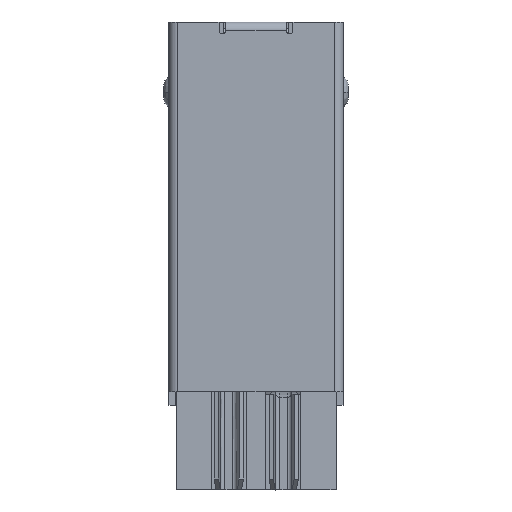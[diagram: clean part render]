
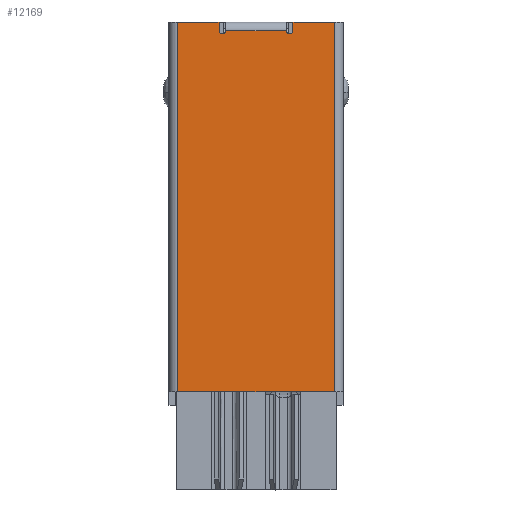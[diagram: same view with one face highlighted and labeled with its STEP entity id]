
A CAD part, front view. The second image highlights one B-rep face of the part: STEP entity #12169.
In plain terms, the highlighted face is planar.
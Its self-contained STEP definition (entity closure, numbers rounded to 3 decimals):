
#36 = CARTESIAN_POINT ( 'NONE',  ( 15.775, 8.618, 0. ) ) ;
#47 = CARTESIAN_POINT ( 'NONE',  ( 15.775, 13.918, -17. ) ) ;
#470 = CARTESIAN_POINT ( 'NONE',  ( 15.775, 12.018, -0.4 ) ) ;
#772 = EDGE_CURVE ( 'NONE', #9003, #23572, #12551, .T. ) ;
#1052 = CARTESIAN_POINT ( 'NONE',  ( 15.775, 10.318, 0. ) ) ;
#1074 = DIRECTION ( 'NONE',  ( -1., 0., 0. ) ) ;
#1161 = VERTEX_POINT ( 'NONE', #36 ) ;
#1164 = DIRECTION ( 'NONE',  ( -1., 0., 0. ) ) ;
#1390 = CARTESIAN_POINT ( 'NONE',  ( 15.775, 10.318, -17. ) ) ;
#1419 = ORIENTED_EDGE ( 'NONE', *, *, #16090, .T. ) ;
#1442 = AXIS2_PLACEMENT_3D ( 'NONE', #2475, #9698, #9934 ) ;
#1840 = DIRECTION ( 'NONE',  ( 1., 0., 0. ) ) ;
#1901 = DIRECTION ( 'NONE',  ( 0., 0., 1. ) ) ;
#1944 = CARTESIAN_POINT ( 'NONE',  ( 15.775, 6.718, -17. ) ) ;
#2215 = CARTESIAN_POINT ( 'NONE',  ( 15.775, 11.718, -0.4 ) ) ;
#2237 = LINE ( 'NONE', #2469, #21916 ) ;
#2265 = EDGE_LOOP ( 'NONE', ( #2969, #20408, #13631, #16832, #23114, #19453, #1419, #18053, #5312, #18673, #3849 ) ) ;
#2469 = CARTESIAN_POINT ( 'NONE',  ( 15.775, 10.318, -0.4 ) ) ;
#2475 = CARTESIAN_POINT ( 'NONE',  ( 15.775, 8.768, -0.4 ) ) ;
#2521 = DIRECTION ( 'NONE',  ( 0., -1., 0. ) ) ;
#2943 = CIRCLE ( 'NONE', #11157, 0.15 ) ;
#2969 = ORIENTED_EDGE ( 'NONE', *, *, #10550, .T. ) ;
#3849 = ORIENTED_EDGE ( 'NONE', *, *, #772, .T. ) ;
#4062 = CARTESIAN_POINT ( 'NONE',  ( 15.775, 6.718, 0. ) ) ;
#4131 = VERTEX_POINT ( 'NONE', #4062 ) ;
#5312 = ORIENTED_EDGE ( 'NONE', *, *, #13490, .T. ) ;
#5510 = CARTESIAN_POINT ( 'NONE',  ( 15.775, 6.568, -17.34 ) ) ;
#5815 = DIRECTION ( 'NONE',  ( 0., -1., 0. ) ) ;
#5989 = LINE ( 'NONE', #21129, #10350 ) ;
#6026 = DIRECTION ( 'NONE',  ( 0., -1., 0. ) ) ;
#6603 = EDGE_CURVE ( 'NONE', #22837, #13406, #2237, .T. ) ;
#6836 = AXIS2_PLACEMENT_3D ( 'NONE', #5510, #1840, #20425 ) ;
#6957 = DIRECTION ( 'NONE',  ( 0., 0., -1. ) ) ;
#7524 = EDGE_CURVE ( 'NONE', #21840, #1161, #18659, .T. ) ;
#7940 = CARTESIAN_POINT ( 'NONE',  ( 15.775, 8.918, -0.4 ) ) ;
#8231 = CARTESIAN_POINT ( 'NONE',  ( 15.775, 6.718, -8.5 ) ) ;
#9003 = VERTEX_POINT ( 'NONE', #9581 ) ;
#9063 = PLANE ( 'NONE',  #6836 ) ;
#9328 = LINE ( 'NONE', #1390, #12747 ) ;
#9367 = VERTEX_POINT ( 'NONE', #14322 ) ;
#9581 = CARTESIAN_POINT ( 'NONE',  ( 15.775, 12.018, 0. ) ) ;
#9698 = DIRECTION ( 'NONE',  ( -1., 0., 0. ) ) ;
#9724 = LINE ( 'NONE', #9962, #23338 ) ;
#9934 = DIRECTION ( 'NONE',  ( 0., 0., -1. ) ) ;
#9962 = CARTESIAN_POINT ( 'NONE',  ( 15.775, 10.318, 0. ) ) ;
#10094 = DIRECTION ( 'NONE',  ( 0., 0., 1. ) ) ;
#10123 = EDGE_CURVE ( 'NONE', #13406, #21769, #15832, .T. ) ;
#10350 = VECTOR ( 'NONE', #13458, 1000. ) ;
#10550 = EDGE_CURVE ( 'NONE', #23572, #22837, #2943, .T. ) ;
#10589 = CARTESIAN_POINT ( 'NONE',  ( 15.775, 11.868, -0.4 ) ) ;
#10834 = VERTEX_POINT ( 'NONE', #47 ) ;
#11126 = VERTEX_POINT ( 'NONE', #1944 ) ;
#11157 = AXIS2_PLACEMENT_3D ( 'NONE', #10589, #1164, #10094 ) ;
#11193 = CARTESIAN_POINT ( 'NONE',  ( 15.775, 8.618, -8.5 ) ) ;
#12169 = ADVANCED_FACE ( 'NONE', ( #12855 ), #9063, .T. ) ;
#12551 = LINE ( 'NONE', #14519, #22301 ) ;
#12747 = VECTOR ( 'NONE', #19978, 1000. ) ;
#12759 = VECTOR ( 'NONE', #19605, 1000. ) ;
#12855 = FACE_OUTER_BOUND ( 'NONE', #2265, .T. ) ;
#13406 = VERTEX_POINT ( 'NONE', #7940 ) ;
#13458 = DIRECTION ( 'NONE',  ( 0., 0., 1. ) ) ;
#13490 = EDGE_CURVE ( 'NONE', #10834, #9367, #5989, .T. ) ;
#13631 = ORIENTED_EDGE ( 'NONE', *, *, #10123, .T. ) ;
#13873 = EDGE_CURVE ( 'NONE', #1161, #4131, #17942, .T. ) ;
#13991 = LINE ( 'NONE', #8231, #12759 ) ;
#14322 = CARTESIAN_POINT ( 'NONE',  ( 15.775, 13.918, 0. ) ) ;
#14416 = CARTESIAN_POINT ( 'NONE',  ( 15.775, 8.768, -0.4 ) ) ;
#14519 = CARTESIAN_POINT ( 'NONE',  ( 15.775, 12.018, -8.5 ) ) ;
#15832 = CIRCLE ( 'NONE', #20953, 0.15 ) ;
#16090 = EDGE_CURVE ( 'NONE', #4131, #11126, #13991, .T. ) ;
#16832 = ORIENTED_EDGE ( 'NONE', *, *, #20488, .T. ) ;
#17942 = LINE ( 'NONE', #1052, #18576 ) ;
#18053 = ORIENTED_EDGE ( 'NONE', *, *, #19460, .T. ) ;
#18576 = VECTOR ( 'NONE', #2521, 1000. ) ;
#18659 = LINE ( 'NONE', #11193, #21466 ) ;
#18673 = ORIENTED_EDGE ( 'NONE', *, *, #21461, .T. ) ;
#19453 = ORIENTED_EDGE ( 'NONE', *, *, #13873, .T. ) ;
#19460 = EDGE_CURVE ( 'NONE', #11126, #10834, #9328, .T. ) ;
#19605 = DIRECTION ( 'NONE',  ( 0., 0., -1. ) ) ;
#19978 = DIRECTION ( 'NONE',  ( 0., 1., 0. ) ) ;
#20008 = DIRECTION ( 'NONE',  ( 0., 0., -1. ) ) ;
#20075 = CARTESIAN_POINT ( 'NONE',  ( 15.775, 8.618, -0.4 ) ) ;
#20408 = ORIENTED_EDGE ( 'NONE', *, *, #6603, .T. ) ;
#20425 = DIRECTION ( 'NONE',  ( 0., 1., 0. ) ) ;
#20488 = EDGE_CURVE ( 'NONE', #21769, #21840, #23712, .T. ) ;
#20953 = AXIS2_PLACEMENT_3D ( 'NONE', #14416, #1074, #6957 ) ;
#21129 = CARTESIAN_POINT ( 'NONE',  ( 15.775, 13.918, -8.5 ) ) ;
#21461 = EDGE_CURVE ( 'NONE', #9367, #9003, #9724, .T. ) ;
#21466 = VECTOR ( 'NONE', #1901, 1000. ) ;
#21769 = VERTEX_POINT ( 'NONE', #23873 ) ;
#21840 = VERTEX_POINT ( 'NONE', #20075 ) ;
#21916 = VECTOR ( 'NONE', #6026, 1000. ) ;
#22301 = VECTOR ( 'NONE', #20008, 1000. ) ;
#22837 = VERTEX_POINT ( 'NONE', #2215 ) ;
#23114 = ORIENTED_EDGE ( 'NONE', *, *, #7524, .T. ) ;
#23338 = VECTOR ( 'NONE', #5815, 1000. ) ;
#23572 = VERTEX_POINT ( 'NONE', #470 ) ;
#23712 = CIRCLE ( 'NONE', #1442, 0.15 ) ;
#23873 = CARTESIAN_POINT ( 'NONE',  ( 15.775, 8.768, -0.55 ) ) ;
